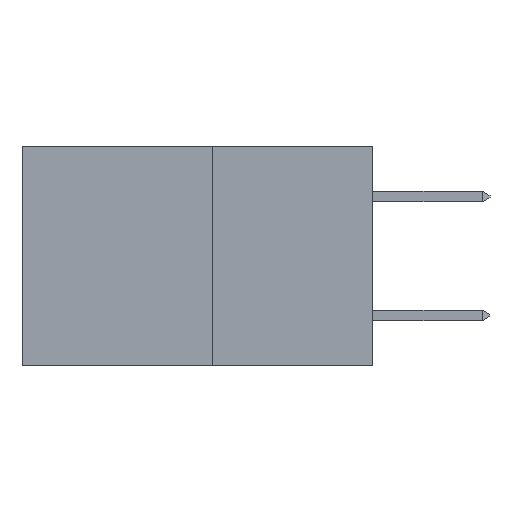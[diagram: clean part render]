
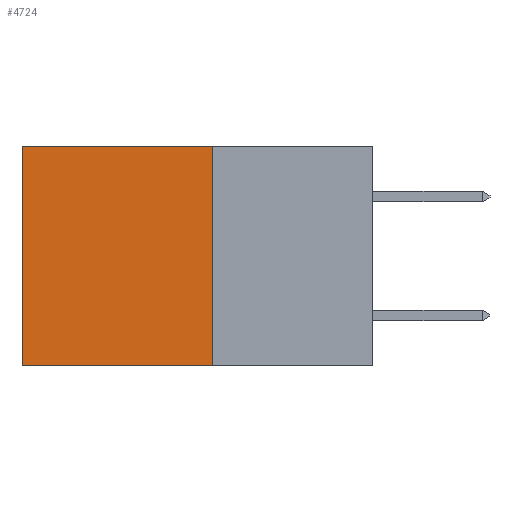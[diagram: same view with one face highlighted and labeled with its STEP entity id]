
A CAD part, left-side view. The second image highlights one B-rep face of the part: STEP entity #4724.
In plain terms, the highlighted planar face has unit normal (-1, 0, 0).
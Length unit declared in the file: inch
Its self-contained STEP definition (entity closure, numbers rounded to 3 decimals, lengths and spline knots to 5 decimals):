
#264 = LINE ( 'NONE', #3046, #6761 ) ;
#456 = ORIENTED_EDGE ( 'NONE', *, *, #6166, .T. ) ;
#709 = VECTOR ( 'NONE', #1887, 39.37008 ) ;
#1198 = LINE ( 'NONE', #6994, #7424 ) ;
#1212 = CARTESIAN_POINT ( 'NONE',  ( 0.277, 0.27, -0.37 ) ) ;
#1264 = VERTEX_POINT ( 'NONE', #1212 ) ;
#1395 = VECTOR ( 'NONE', #1912, 39.37008 ) ;
#1562 = ORIENTED_EDGE ( 'NONE', *, *, #4475, .F. ) ;
#1887 = DIRECTION ( 'NONE',  ( 0., 1., 0. ) ) ;
#1889 = CARTESIAN_POINT ( 'NONE',  ( 0.277, 0.27, 0. ) ) ;
#1912 = DIRECTION ( 'NONE',  ( 0., 1., 0. ) ) ;
#1991 = CARTESIAN_POINT ( 'NONE',  ( 0.277, 0.27, -0.37 ) ) ;
#2613 = ORIENTED_EDGE ( 'NONE', *, *, #6275, .F. ) ;
#2840 = DIRECTION ( 'NONE',  ( 0., 0., -1. ) ) ;
#3046 = CARTESIAN_POINT ( 'NONE',  ( 0.277, 0.59, -0.37 ) ) ;
#3099 = LINE ( 'NONE', #1991, #1395 ) ;
#3549 = VERTEX_POINT ( 'NONE', #7481 ) ;
#4089 = LINE ( 'NONE', #1889, #709 ) ;
#4475 = EDGE_CURVE ( 'NONE', #7709, #1264, #1198, .T. ) ;
#4518 = AXIS2_PLACEMENT_3D ( 'NONE', #5457, #5396, #5394 ) ;
#4724 = ADVANCED_FACE ( 'NONE', ( #6510 ), #5406, .F. ) ;
#4809 = ORIENTED_EDGE ( 'NONE', *, *, #5211, .T. ) ;
#5012 = CARTESIAN_POINT ( 'NONE',  ( 0.277, 0.59, 0. ) ) ;
#5211 = EDGE_CURVE ( 'NONE', #7709, #6055, #4089, .T. ) ;
#5388 = CARTESIAN_POINT ( 'NONE',  ( 0.277, 0.27, 0. ) ) ;
#5394 = DIRECTION ( 'NONE',  ( 0., 0., -1. ) ) ;
#5396 = DIRECTION ( 'NONE',  ( 1., 0., 0. ) ) ;
#5406 = PLANE ( 'NONE',  #4518 ) ;
#5457 = CARTESIAN_POINT ( 'NONE',  ( 0.277, 0.27, -0.37 ) ) ;
#6055 = VERTEX_POINT ( 'NONE', #5012 ) ;
#6166 = EDGE_CURVE ( 'NONE', #6055, #3549, #264, .T. ) ;
#6275 = EDGE_CURVE ( 'NONE', #1264, #3549, #3099, .T. ) ;
#6510 = FACE_OUTER_BOUND ( 'NONE', #7491, .T. ) ;
#6761 = VECTOR ( 'NONE', #2840, 39.37008 ) ;
#6986 = DIRECTION ( 'NONE',  ( 0., 0., -1. ) ) ;
#6994 = CARTESIAN_POINT ( 'NONE',  ( 0.277, 0.27, -0.37 ) ) ;
#7424 = VECTOR ( 'NONE', #6986, 39.37008 ) ;
#7481 = CARTESIAN_POINT ( 'NONE',  ( 0.277, 0.59, -0.37 ) ) ;
#7491 = EDGE_LOOP ( 'NONE', ( #456, #2613, #1562, #4809 ) ) ;
#7709 = VERTEX_POINT ( 'NONE', #5388 ) ;
